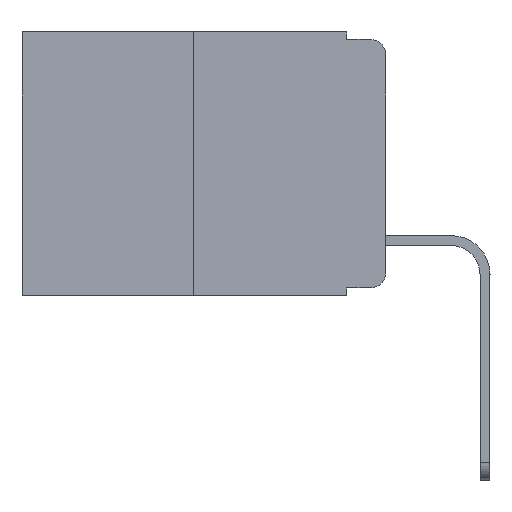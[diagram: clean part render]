
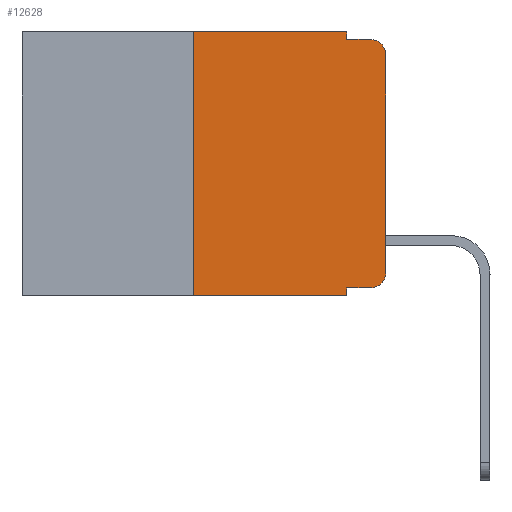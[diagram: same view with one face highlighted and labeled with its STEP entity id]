
A CAD part, left-side view. The second image highlights one B-rep face of the part: STEP entity #12628.
In plain terms, the highlighted planar face has unit normal (-1, 0, 0).
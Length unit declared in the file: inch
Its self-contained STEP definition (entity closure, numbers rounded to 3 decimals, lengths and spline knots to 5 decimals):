
#313 = ORIENTED_EDGE ( 'NONE', *, *, #2484, .T. ) ;
#443 = DIRECTION ( 'NONE',  ( -1., 0., 0. ) ) ;
#815 = VECTOR ( 'NONE', #10519, 39.37008 ) ;
#841 = VERTEX_POINT ( 'NONE', #1178 ) ;
#969 = CARTESIAN_POINT ( 'NONE',  ( 0., 0.051, -0.343 ) ) ;
#1178 = CARTESIAN_POINT ( 'NONE',  ( 0., 0.051, -0.333 ) ) ;
#1180 = CARTESIAN_POINT ( 'NONE',  ( 0., 0.473, 0. ) ) ;
#1311 = EDGE_CURVE ( 'NONE', #4255, #7053, #1741, .T. ) ;
#1741 = LINE ( 'NONE', #9841, #12129 ) ;
#1815 = VERTEX_POINT ( 'NONE', #2155 ) ;
#2039 = CARTESIAN_POINT ( 'NONE',  ( 0., 0., 0. ) ) ;
#2155 = CARTESIAN_POINT ( 'NONE',  ( 0., 0.02, -0.333 ) ) ;
#2278 = DIRECTION ( 'NONE',  ( 0., -1., 0. ) ) ;
#2484 = EDGE_CURVE ( 'NONE', #2977, #13293, #11722, .T. ) ;
#2554 = CARTESIAN_POINT ( 'NONE',  ( 0., 0.051, -0.01 ) ) ;
#2560 = VECTOR ( 'NONE', #5513, 39.37008 ) ;
#2773 = ORIENTED_EDGE ( 'NONE', *, *, #4045, .F. ) ;
#2862 = CARTESIAN_POINT ( 'NONE',  ( 0., 0.02, -0.313 ) ) ;
#2935 = EDGE_CURVE ( 'NONE', #1815, #2977, #14201, .T. ) ;
#2977 = VERTEX_POINT ( 'NONE', #11636 ) ;
#3124 = LINE ( 'NONE', #9200, #2560 ) ;
#3184 = CARTESIAN_POINT ( 'NONE',  ( 0., 0.051, 0. ) ) ;
#3548 = EDGE_CURVE ( 'NONE', #8555, #11777, #3124, .T. ) ;
#3808 = ORIENTED_EDGE ( 'NONE', *, *, #1311, .F. ) ;
#3812 = ORIENTED_EDGE ( 'NONE', *, *, #3548, .F. ) ;
#3975 = FACE_OUTER_BOUND ( 'NONE', #9740, .T. ) ;
#4045 = EDGE_CURVE ( 'NONE', #841, #11049, #4448, .T. ) ;
#4255 = VERTEX_POINT ( 'NONE', #11429 ) ;
#4372 = VECTOR ( 'NONE', #4474, 39.37008 ) ;
#4448 = LINE ( 'NONE', #3184, #815 ) ;
#4474 = DIRECTION ( 'NONE',  ( 0., 0., 1. ) ) ;
#4583 = CARTESIAN_POINT ( 'NONE',  ( 0., 0.25, 0. ) ) ;
#4830 = AXIS2_PLACEMENT_3D ( 'NONE', #13025, #14279, #6901 ) ;
#4936 = AXIS2_PLACEMENT_3D ( 'NONE', #1180, #8352, #10867 ) ;
#5513 = DIRECTION ( 'NONE',  ( 0., -1., 0. ) ) ;
#5762 = ORIENTED_EDGE ( 'NONE', *, *, #13212, .F. ) ;
#5848 = LINE ( 'NONE', #13105, #15718 ) ;
#6272 = VECTOR ( 'NONE', #14984, 39.37008 ) ;
#6901 = DIRECTION ( 'NONE',  ( 0., 0., -1. ) ) ;
#7053 = VERTEX_POINT ( 'NONE', #11890 ) ;
#7806 = EDGE_CURVE ( 'NONE', #8727, #11049, #10727, .T. ) ;
#8352 = DIRECTION ( 'NONE',  ( 1., 0., 0. ) ) ;
#8389 = DIRECTION ( 'NONE',  ( 0., 0., -1. ) ) ;
#8460 = VECTOR ( 'NONE', #10706, 39.37008 ) ;
#8492 = EDGE_CURVE ( 'NONE', #841, #1815, #5848, .T. ) ;
#8493 = ORIENTED_EDGE ( 'NONE', *, *, #2935, .T. ) ;
#8555 = VERTEX_POINT ( 'NONE', #2554 ) ;
#8688 = ORIENTED_EDGE ( 'NONE', *, *, #7806, .T. ) ;
#8727 = VERTEX_POINT ( 'NONE', #10008 ) ;
#9200 = CARTESIAN_POINT ( 'NONE',  ( 0., 0.051, -0.01 ) ) ;
#9740 = EDGE_LOOP ( 'NONE', ( #313, #15921, #3812, #5762, #3808, #14583, #8688, #2773, #10046, #8493 ) ) ;
#9797 = CARTESIAN_POINT ( 'NONE',  ( 0., 0., -0.03 ) ) ;
#9841 = CARTESIAN_POINT ( 'NONE',  ( 0., 0.473, 0. ) ) ;
#10008 = CARTESIAN_POINT ( 'NONE',  ( 0., 0.25, -0.343 ) ) ;
#10046 = ORIENTED_EDGE ( 'NONE', *, *, #8492, .T. ) ;
#10064 = CARTESIAN_POINT ( 'NONE',  ( 0., 0.473, -0.343 ) ) ;
#10509 = CIRCLE ( 'NONE', #4830, 0.02 ) ;
#10519 = DIRECTION ( 'NONE',  ( 0., 0., -1. ) ) ;
#10643 = CARTESIAN_POINT ( 'NONE',  ( 0., 0.051, 0. ) ) ;
#10706 = DIRECTION ( 'NONE',  ( 0., 0., 1. ) ) ;
#10727 = LINE ( 'NONE', #10064, #6272 ) ;
#10867 = DIRECTION ( 'NONE',  ( 0., 0., -1. ) ) ;
#11049 = VERTEX_POINT ( 'NONE', #969 ) ;
#11155 = LINE ( 'NONE', #10643, #15786 ) ;
#11429 = CARTESIAN_POINT ( 'NONE',  ( 0., 0.25, 0. ) ) ;
#11473 = DIRECTION ( 'NONE',  ( 0., 0., -1. ) ) ;
#11636 = CARTESIAN_POINT ( 'NONE',  ( 0., 0., -0.313 ) ) ;
#11722 = LINE ( 'NONE', #2039, #8460 ) ;
#11777 = VERTEX_POINT ( 'NONE', #15149 ) ;
#11890 = CARTESIAN_POINT ( 'NONE',  ( 0., 0.051, 0. ) ) ;
#12129 = VECTOR ( 'NONE', #2278, 39.37008 ) ;
#12628 = ADVANCED_FACE ( 'NONE', ( #3975 ), #13332, .F. ) ;
#13025 = CARTESIAN_POINT ( 'NONE',  ( 0., 0.02, -0.03 ) ) ;
#13105 = CARTESIAN_POINT ( 'NONE',  ( 0., 0.051, -0.333 ) ) ;
#13212 = EDGE_CURVE ( 'NONE', #7053, #8555, #11155, .T. ) ;
#13217 = EDGE_CURVE ( 'NONE', #8727, #4255, #14979, .T. ) ;
#13293 = VERTEX_POINT ( 'NONE', #9797 ) ;
#13332 = PLANE ( 'NONE',  #4936 ) ;
#14201 = CIRCLE ( 'NONE', #15907, 0.02 ) ;
#14279 = DIRECTION ( 'NONE',  ( -1., 0., 0. ) ) ;
#14392 = DIRECTION ( 'NONE',  ( 0., -1., 0. ) ) ;
#14583 = ORIENTED_EDGE ( 'NONE', *, *, #13217, .F. ) ;
#14649 = EDGE_CURVE ( 'NONE', #13293, #11777, #10509, .T. ) ;
#14979 = LINE ( 'NONE', #4583, #4372 ) ;
#14984 = DIRECTION ( 'NONE',  ( 0., -1., 0. ) ) ;
#15149 = CARTESIAN_POINT ( 'NONE',  ( 0., 0.02, -0.01 ) ) ;
#15718 = VECTOR ( 'NONE', #14392, 39.37008 ) ;
#15786 = VECTOR ( 'NONE', #8389, 39.37008 ) ;
#15907 = AXIS2_PLACEMENT_3D ( 'NONE', #2862, #443, #11473 ) ;
#15921 = ORIENTED_EDGE ( 'NONE', *, *, #14649, .T. ) ;
